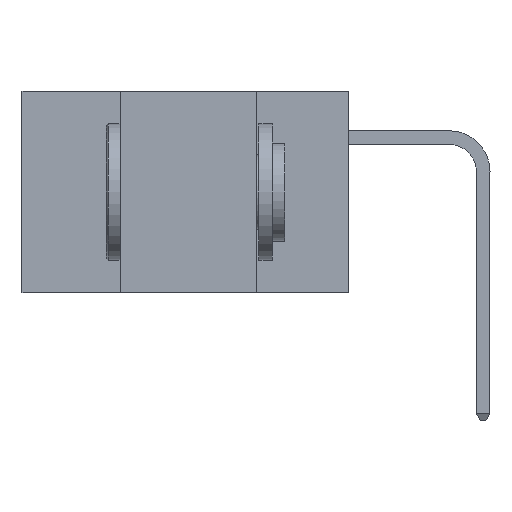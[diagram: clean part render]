
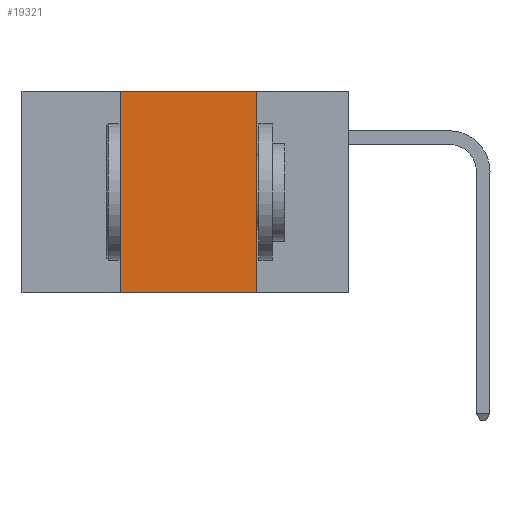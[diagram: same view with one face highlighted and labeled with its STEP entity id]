
A CAD part, left-side view. The second image highlights one B-rep face of the part: STEP entity #19321.
In plain terms, the highlighted planar face has unit normal (-1, 0, 0).
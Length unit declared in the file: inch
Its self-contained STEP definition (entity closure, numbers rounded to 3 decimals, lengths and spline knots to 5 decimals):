
#3063 = ORIENTED_EDGE ( 'NONE', *, *, #16060, .T. ) ;
#3501 = VECTOR ( 'NONE', #19598, 39.37008 ) ;
#3880 = CARTESIAN_POINT ( 'NONE',  ( 0., 0.6, 0. ) ) ;
#3959 = VERTEX_POINT ( 'NONE', #11089 ) ;
#4015 = VECTOR ( 'NONE', #4045, 39.37008 ) ;
#4045 = DIRECTION ( 'NONE',  ( 0., -1., 0. ) ) ;
#4407 = EDGE_LOOP ( 'NONE', ( #17659, #5569, #9992, #3063 ) ) ;
#4691 = CARTESIAN_POINT ( 'NONE',  ( 0., 0.17, -0.37 ) ) ;
#5569 = ORIENTED_EDGE ( 'NONE', *, *, #11118, .F. ) ;
#5773 = CARTESIAN_POINT ( 'NONE',  ( 0., 0.42, 0. ) ) ;
#5777 = VERTEX_POINT ( 'NONE', #4691 ) ;
#5906 = DIRECTION ( 'NONE',  ( 0., 0., -1. ) ) ;
#6191 = CARTESIAN_POINT ( 'NONE',  ( 0., 0.17, 0. ) ) ;
#6270 = CARTESIAN_POINT ( 'NONE',  ( 0., 0.42, -0.37 ) ) ;
#8207 = DIRECTION ( 'NONE',  ( 0., 0., -1. ) ) ;
#8731 = CARTESIAN_POINT ( 'NONE',  ( 0., 0.42, 0. ) ) ;
#9992 = ORIENTED_EDGE ( 'NONE', *, *, #15079, .F. ) ;
#11089 = CARTESIAN_POINT ( 'NONE',  ( 0., 0.17, 0. ) ) ;
#11118 = EDGE_CURVE ( 'NONE', #13590, #3959, #19823, .T. ) ;
#13590 = VERTEX_POINT ( 'NONE', #8731 ) ;
#14586 = DIRECTION ( 'NONE',  ( 0., -1., 0. ) ) ;
#15079 = EDGE_CURVE ( 'NONE', #22479, #13590, #18696, .T. ) ;
#15976 = AXIS2_PLACEMENT_3D ( 'NONE', #3880, #17768, #5906 ) ;
#16060 = EDGE_CURVE ( 'NONE', #22479, #5777, #21398, .T. ) ;
#16995 = VECTOR ( 'NONE', #8207, 39.37008 ) ;
#17659 = ORIENTED_EDGE ( 'NONE', *, *, #24246, .F. ) ;
#17768 = DIRECTION ( 'NONE',  ( 1., 0., 0. ) ) ;
#17949 = CARTESIAN_POINT ( 'NONE',  ( 0., 0.6, 0. ) ) ;
#18473 = FACE_OUTER_BOUND ( 'NONE', #4407, .T. ) ;
#18696 = LINE ( 'NONE', #5773, #3501 ) ;
#19321 = ADVANCED_FACE ( 'NONE', ( #18473 ), #23561, .F. ) ;
#19598 = DIRECTION ( 'NONE',  ( 0., 0., 1. ) ) ;
#19823 = LINE ( 'NONE', #17949, #4015 ) ;
#20767 = VECTOR ( 'NONE', #14586, 39.37008 ) ;
#21398 = LINE ( 'NONE', #24386, #20767 ) ;
#22200 = LINE ( 'NONE', #6191, #16995 ) ;
#22479 = VERTEX_POINT ( 'NONE', #6270 ) ;
#23561 = PLANE ( 'NONE',  #15976 ) ;
#24246 = EDGE_CURVE ( 'NONE', #3959, #5777, #22200, .T. ) ;
#24386 = CARTESIAN_POINT ( 'NONE',  ( 0., 0.6, -0.37 ) ) ;
